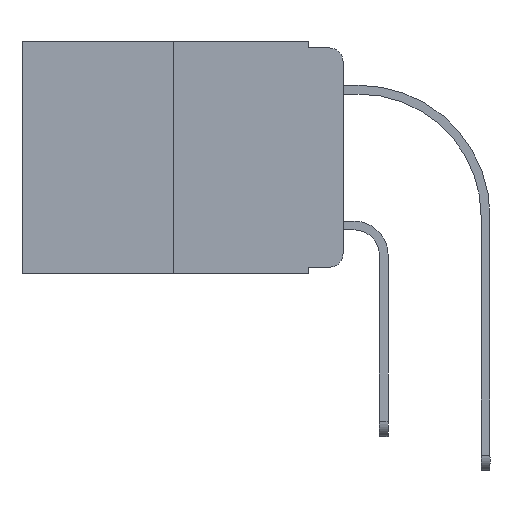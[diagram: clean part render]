
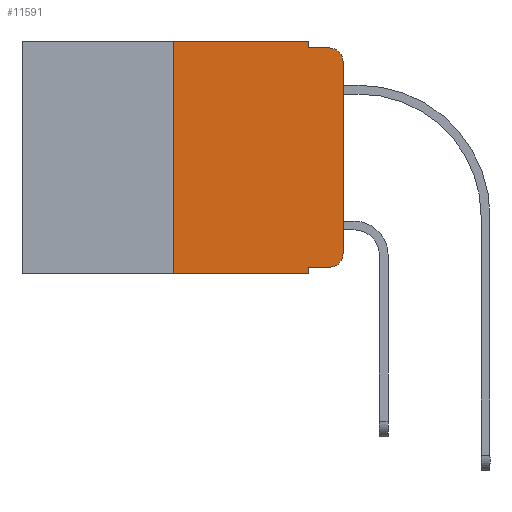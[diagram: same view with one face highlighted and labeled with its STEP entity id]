
A CAD part, left-side view. The second image highlights one B-rep face of the part: STEP entity #11591.
In plain terms, the highlighted planar face has unit normal (-1, 0, 0).
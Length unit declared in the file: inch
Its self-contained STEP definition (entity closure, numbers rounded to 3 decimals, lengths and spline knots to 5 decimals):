
#47 = CARTESIAN_POINT ( 'NONE',  ( 0., 0.25, -0.343 ) ) ;
#113 = LINE ( 'NONE', #6840, #315 ) ;
#128 = DIRECTION ( 'NONE',  ( 0., 0., -1. ) ) ;
#291 = VECTOR ( 'NONE', #6175, 39.37008 ) ;
#311 = ORIENTED_EDGE ( 'NONE', *, *, #5702, .F. ) ;
#315 = VECTOR ( 'NONE', #7842, 39.37008 ) ;
#351 = EDGE_CURVE ( 'NONE', #2103, #4962, #7689, .T. ) ;
#416 = DIRECTION ( 'NONE',  ( 0., 0., -1. ) ) ;
#540 = FACE_OUTER_BOUND ( 'NONE', #5601, .T. ) ;
#633 = LINE ( 'NONE', #7410, #5173 ) ;
#823 = LINE ( 'NONE', #2886, #11019 ) ;
#917 = DIRECTION ( 'NONE',  ( 0., -1., 0. ) ) ;
#1004 = VERTEX_POINT ( 'NONE', #8169 ) ;
#1388 = CIRCLE ( 'NONE', #10008, 0.02 ) ;
#1683 = LINE ( 'NONE', #5920, #8206 ) ;
#1988 = VERTEX_POINT ( 'NONE', #4822 ) ;
#2001 = DIRECTION ( 'NONE',  ( 0., -1., 0. ) ) ;
#2095 = CARTESIAN_POINT ( 'NONE',  ( 0., 0.051, -0.01 ) ) ;
#2103 = VERTEX_POINT ( 'NONE', #9948 ) ;
#2358 = CARTESIAN_POINT ( 'NONE',  ( 0., 0., -0.03 ) ) ;
#2391 = ORIENTED_EDGE ( 'NONE', *, *, #11772, .T. ) ;
#2393 = CARTESIAN_POINT ( 'NONE',  ( 0., 0., -0.313 ) ) ;
#2490 = CARTESIAN_POINT ( 'NONE',  ( 0., 0.473, 0. ) ) ;
#2631 = VERTEX_POINT ( 'NONE', #2393 ) ;
#2824 = VERTEX_POINT ( 'NONE', #3707 ) ;
#2886 = CARTESIAN_POINT ( 'NONE',  ( 0., 0.473, -0.343 ) ) ;
#2973 = DIRECTION ( 'NONE',  ( 0., 0., 1. ) ) ;
#2984 = AXIS2_PLACEMENT_3D ( 'NONE', #2490, #10963, #416 ) ;
#3287 = ORIENTED_EDGE ( 'NONE', *, *, #5940, .T. ) ;
#3300 = EDGE_CURVE ( 'NONE', #11680, #4962, #1388, .T. ) ;
#3475 = EDGE_CURVE ( 'NONE', #9635, #1988, #10609, .T. ) ;
#3593 = ORIENTED_EDGE ( 'NONE', *, *, #8342, .F. ) ;
#3707 = CARTESIAN_POINT ( 'NONE',  ( 0., 0.051, -0.343 ) ) ;
#3730 = LINE ( 'NONE', #11650, #9841 ) ;
#3757 = DIRECTION ( 'NONE',  ( 0., 0., 1. ) ) ;
#4090 = CARTESIAN_POINT ( 'NONE',  ( 0., 0.473, 0. ) ) ;
#4822 = CARTESIAN_POINT ( 'NONE',  ( 0., 0.051, 0. ) ) ;
#4962 = VERTEX_POINT ( 'NONE', #8353 ) ;
#5029 = CARTESIAN_POINT ( 'NONE',  ( 0., 0.02, -0.313 ) ) ;
#5173 = VECTOR ( 'NONE', #3757, 39.37008 ) ;
#5601 = EDGE_LOOP ( 'NONE', ( #9040, #8910, #6141, #8286, #9450, #3593, #7630, #311, #2391, #3287 ) ) ;
#5702 = EDGE_CURVE ( 'NONE', #1004, #2824, #6430, .T. ) ;
#5920 = CARTESIAN_POINT ( 'NONE',  ( 0., 0.051, -0.333 ) ) ;
#5940 = EDGE_CURVE ( 'NONE', #9234, #2631, #8930, .T. ) ;
#6141 = ORIENTED_EDGE ( 'NONE', *, *, #351, .F. ) ;
#6175 = DIRECTION ( 'NONE',  ( 0., -1., 0. ) ) ;
#6301 = DIRECTION ( 'NONE',  ( 0., 0., -1. ) ) ;
#6405 = EDGE_CURVE ( 'NONE', #1988, #2103, #113, .T. ) ;
#6430 = LINE ( 'NONE', #12196, #8531 ) ;
#6840 = CARTESIAN_POINT ( 'NONE',  ( 0., 0.051, 0. ) ) ;
#7410 = CARTESIAN_POINT ( 'NONE',  ( 0., 0.25, 0. ) ) ;
#7630 = ORIENTED_EDGE ( 'NONE', *, *, #12161, .T. ) ;
#7689 = LINE ( 'NONE', #2095, #291 ) ;
#7842 = DIRECTION ( 'NONE',  ( 0., 0., -1. ) ) ;
#7858 = DIRECTION ( 'NONE',  ( -1., 0., 0. ) ) ;
#8169 = CARTESIAN_POINT ( 'NONE',  ( 0., 0.051, -0.333 ) ) ;
#8206 = VECTOR ( 'NONE', #917, 39.37008 ) ;
#8286 = ORIENTED_EDGE ( 'NONE', *, *, #6405, .F. ) ;
#8342 = EDGE_CURVE ( 'NONE', #11536, #9635, #633, .T. ) ;
#8353 = CARTESIAN_POINT ( 'NONE',  ( 0., 0.02, -0.01 ) ) ;
#8447 = CARTESIAN_POINT ( 'NONE',  ( 0., 0.02, -0.333 ) ) ;
#8531 = VECTOR ( 'NONE', #6301, 39.37008 ) ;
#8604 = VECTOR ( 'NONE', #9608, 39.37008 ) ;
#8910 = ORIENTED_EDGE ( 'NONE', *, *, #3300, .T. ) ;
#8930 = CIRCLE ( 'NONE', #11948, 0.02 ) ;
#9023 = PLANE ( 'NONE',  #2984 ) ;
#9040 = ORIENTED_EDGE ( 'NONE', *, *, #9436, .T. ) ;
#9234 = VERTEX_POINT ( 'NONE', #8447 ) ;
#9308 = DIRECTION ( 'NONE',  ( 0., 0., -1. ) ) ;
#9436 = EDGE_CURVE ( 'NONE', #2631, #11680, #3730, .T. ) ;
#9450 = ORIENTED_EDGE ( 'NONE', *, *, #3475, .F. ) ;
#9608 = DIRECTION ( 'NONE',  ( 0., -1., 0. ) ) ;
#9635 = VERTEX_POINT ( 'NONE', #11831 ) ;
#9841 = VECTOR ( 'NONE', #2973, 39.37008 ) ;
#9948 = CARTESIAN_POINT ( 'NONE',  ( 0., 0.051, -0.01 ) ) ;
#10008 = AXIS2_PLACEMENT_3D ( 'NONE', #12317, #11314, #9308 ) ;
#10609 = LINE ( 'NONE', #4090, #8604 ) ;
#10963 = DIRECTION ( 'NONE',  ( 1., 0., 0. ) ) ;
#11019 = VECTOR ( 'NONE', #2001, 39.37008 ) ;
#11314 = DIRECTION ( 'NONE',  ( -1., 0., 0. ) ) ;
#11536 = VERTEX_POINT ( 'NONE', #47 ) ;
#11591 = ADVANCED_FACE ( 'NONE', ( #540 ), #9023, .F. ) ;
#11650 = CARTESIAN_POINT ( 'NONE',  ( 0., 0., 0. ) ) ;
#11680 = VERTEX_POINT ( 'NONE', #2358 ) ;
#11772 = EDGE_CURVE ( 'NONE', #1004, #9234, #1683, .T. ) ;
#11831 = CARTESIAN_POINT ( 'NONE',  ( 0., 0.25, 0. ) ) ;
#11948 = AXIS2_PLACEMENT_3D ( 'NONE', #5029, #7858, #128 ) ;
#12161 = EDGE_CURVE ( 'NONE', #11536, #2824, #823, .T. ) ;
#12196 = CARTESIAN_POINT ( 'NONE',  ( 0., 0.051, 0. ) ) ;
#12317 = CARTESIAN_POINT ( 'NONE',  ( 0., 0.02, -0.03 ) ) ;
